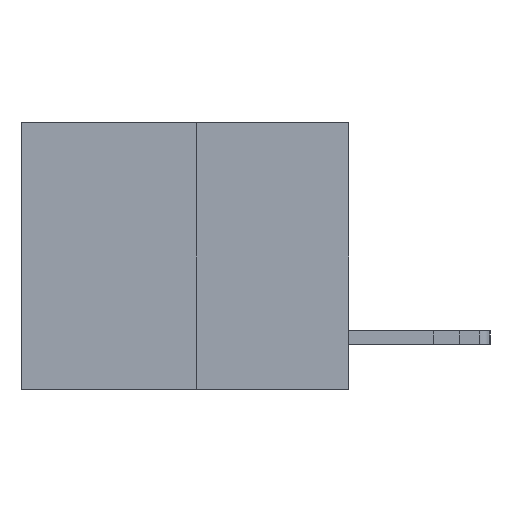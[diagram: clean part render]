
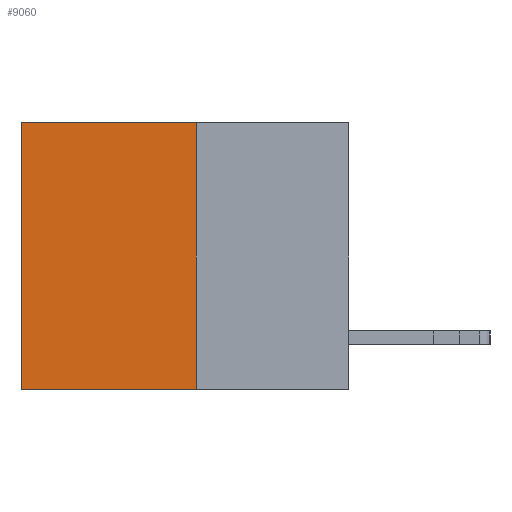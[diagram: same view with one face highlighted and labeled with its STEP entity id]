
A CAD part, left-side view. The second image highlights one B-rep face of the part: STEP entity #9060.
In plain terms, the highlighted planar face has unit normal (-1, 0, 0).
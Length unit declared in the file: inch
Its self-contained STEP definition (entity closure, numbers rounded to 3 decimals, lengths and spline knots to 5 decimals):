
#332 = CARTESIAN_POINT ( 'NONE',  ( 0.3165, 0.28, -0.49 ) ) ;
#984 = CARTESIAN_POINT ( 'NONE',  ( 0.3165, 0.6, -0.49 ) ) ;
#1393 = CARTESIAN_POINT ( 'NONE',  ( 0.3165, 0.28, 0. ) ) ;
#1933 = FACE_OUTER_BOUND ( 'NONE', #3031, .T. ) ;
#2441 = DIRECTION ( 'NONE',  ( 1., 0., 0. ) ) ;
#2796 = LINE ( 'NONE', #10214, #3101 ) ;
#2881 = VERTEX_POINT ( 'NONE', #9735 ) ;
#3031 = EDGE_LOOP ( 'NONE', ( #9733, #9846, #8135, #9252 ) ) ;
#3101 = VECTOR ( 'NONE', #4489, 39.37008 ) ;
#3104 = VECTOR ( 'NONE', #11404, 39.37008 ) ;
#3333 = EDGE_CURVE ( 'NONE', #3787, #7220, #5597, .T. ) ;
#3787 = VERTEX_POINT ( 'NONE', #1393 ) ;
#3934 = VECTOR ( 'NONE', #4757, 39.37008 ) ;
#4037 = CARTESIAN_POINT ( 'NONE',  ( 0.3165, 0.28, 0. ) ) ;
#4489 = DIRECTION ( 'NONE',  ( 0., 1., 0. ) ) ;
#4757 = DIRECTION ( 'NONE',  ( 0., 0., -1. ) ) ;
#5281 = DIRECTION ( 'NONE',  ( 0., 0., -1. ) ) ;
#5597 = LINE ( 'NONE', #6610, #3104 ) ;
#6535 = AXIS2_PLACEMENT_3D ( 'NONE', #7989, #2441, #5281 ) ;
#6610 = CARTESIAN_POINT ( 'NONE',  ( 0.3165, 0.28, -0.49 ) ) ;
#6636 = VECTOR ( 'NONE', #7805, 39.37008 ) ;
#7220 = VERTEX_POINT ( 'NONE', #332 ) ;
#7450 = CARTESIAN_POINT ( 'NONE',  ( 0.3165, 0.6, -0.49 ) ) ;
#7518 = VERTEX_POINT ( 'NONE', #7450 ) ;
#7805 = DIRECTION ( 'NONE',  ( 0., 1., 0. ) ) ;
#7989 = CARTESIAN_POINT ( 'NONE',  ( 0.3165, 0.28, -0.49 ) ) ;
#8113 = LINE ( 'NONE', #4037, #6636 ) ;
#8135 = ORIENTED_EDGE ( 'NONE', *, *, #3333, .F. ) ;
#8583 = EDGE_CURVE ( 'NONE', #3787, #2881, #8113, .T. ) ;
#8912 = LINE ( 'NONE', #984, #3934 ) ;
#8964 = PLANE ( 'NONE',  #6535 ) ;
#9060 = ADVANCED_FACE ( 'NONE', ( #1933 ), #8964, .F. ) ;
#9252 = ORIENTED_EDGE ( 'NONE', *, *, #8583, .T. ) ;
#9733 = ORIENTED_EDGE ( 'NONE', *, *, #11705, .T. ) ;
#9735 = CARTESIAN_POINT ( 'NONE',  ( 0.3165, 0.6, 0. ) ) ;
#9846 = ORIENTED_EDGE ( 'NONE', *, *, #9872, .F. ) ;
#9872 = EDGE_CURVE ( 'NONE', #7220, #7518, #2796, .T. ) ;
#10214 = CARTESIAN_POINT ( 'NONE',  ( 0.3165, 0.28, -0.49 ) ) ;
#11404 = DIRECTION ( 'NONE',  ( 0., 0., -1. ) ) ;
#11705 = EDGE_CURVE ( 'NONE', #2881, #7518, #8912, .T. ) ;
